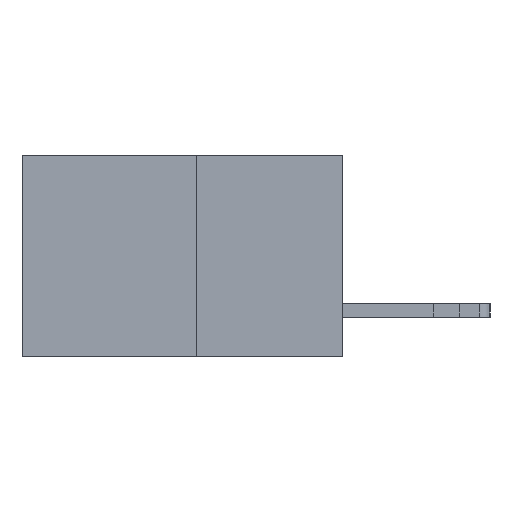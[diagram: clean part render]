
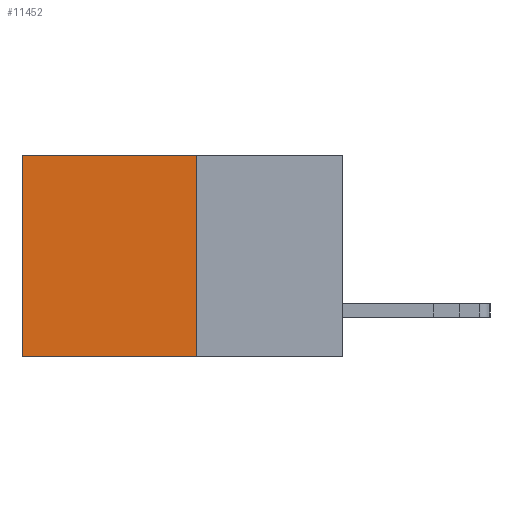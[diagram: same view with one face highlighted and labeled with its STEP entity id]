
A CAD part, left-side view. The second image highlights one B-rep face of the part: STEP entity #11452.
In plain terms, the highlighted planar face has unit normal (-1, 0, 0).
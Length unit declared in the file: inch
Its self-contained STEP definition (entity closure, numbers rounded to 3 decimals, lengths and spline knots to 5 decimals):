
#77 = CARTESIAN_POINT ( 'NONE',  ( 0.277, 0.59, 0. ) ) ;
#210 = VERTEX_POINT ( 'NONE', #11595 ) ;
#748 = ORIENTED_EDGE ( 'NONE', *, *, #7108, .T. ) ;
#797 = DIRECTION ( 'NONE',  ( 0., 1., 0. ) ) ;
#851 = CARTESIAN_POINT ( 'NONE',  ( 0.277, 0.27, -0.37 ) ) ;
#1117 = ORIENTED_EDGE ( 'NONE', *, *, #13645, .F. ) ;
#1604 = VERTEX_POINT ( 'NONE', #11842 ) ;
#1618 = LINE ( 'NONE', #2517, #4154 ) ;
#1663 = DIRECTION ( 'NONE',  ( 0., 1., 0. ) ) ;
#2017 = DIRECTION ( 'NONE',  ( 0., 0., -1. ) ) ;
#2204 = AXIS2_PLACEMENT_3D ( 'NONE', #851, #8499, #2017 ) ;
#2517 = CARTESIAN_POINT ( 'NONE',  ( 0.277, 0.27, -0.37 ) ) ;
#3040 = VERTEX_POINT ( 'NONE', #3611 ) ;
#3611 = CARTESIAN_POINT ( 'NONE',  ( 0.277, 0.27, -0.37 ) ) ;
#4011 = FACE_OUTER_BOUND ( 'NONE', #11832, .T. ) ;
#4154 = VECTOR ( 'NONE', #11113, 39.37008 ) ;
#4451 = VECTOR ( 'NONE', #797, 39.37008 ) ;
#4722 = ORIENTED_EDGE ( 'NONE', *, *, #12041, .F. ) ;
#4801 = DIRECTION ( 'NONE',  ( 0., 0., -1. ) ) ;
#4831 = CARTESIAN_POINT ( 'NONE',  ( 0.277, 0.59, -0.37 ) ) ;
#5407 = VECTOR ( 'NONE', #4801, 39.37008 ) ;
#6317 = CARTESIAN_POINT ( 'NONE',  ( 0.277, 0.27, 0. ) ) ;
#6366 = PLANE ( 'NONE',  #2204 ) ;
#7108 = EDGE_CURVE ( 'NONE', #13444, #210, #11098, .T. ) ;
#7957 = ORIENTED_EDGE ( 'NONE', *, *, #9635, .T. ) ;
#8175 = CARTESIAN_POINT ( 'NONE',  ( 0.277, 0.27, -0.37 ) ) ;
#8499 = DIRECTION ( 'NONE',  ( 1., 0., 0. ) ) ;
#9635 = EDGE_CURVE ( 'NONE', #1604, #13444, #12621, .T. ) ;
#10519 = LINE ( 'NONE', #8175, #12930 ) ;
#11098 = LINE ( 'NONE', #4831, #5407 ) ;
#11113 = DIRECTION ( 'NONE',  ( 0., 0., -1. ) ) ;
#11452 = ADVANCED_FACE ( 'NONE', ( #4011 ), #6366, .F. ) ;
#11595 = CARTESIAN_POINT ( 'NONE',  ( 0.277, 0.59, -0.37 ) ) ;
#11832 = EDGE_LOOP ( 'NONE', ( #748, #1117, #4722, #7957 ) ) ;
#11842 = CARTESIAN_POINT ( 'NONE',  ( 0.277, 0.27, 0. ) ) ;
#12041 = EDGE_CURVE ( 'NONE', #1604, #3040, #1618, .T. ) ;
#12621 = LINE ( 'NONE', #6317, #4451 ) ;
#12930 = VECTOR ( 'NONE', #1663, 39.37008 ) ;
#13444 = VERTEX_POINT ( 'NONE', #77 ) ;
#13645 = EDGE_CURVE ( 'NONE', #3040, #210, #10519, .T. ) ;
